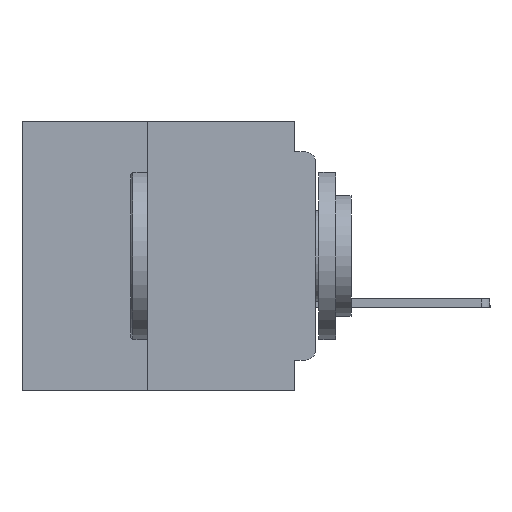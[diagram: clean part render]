
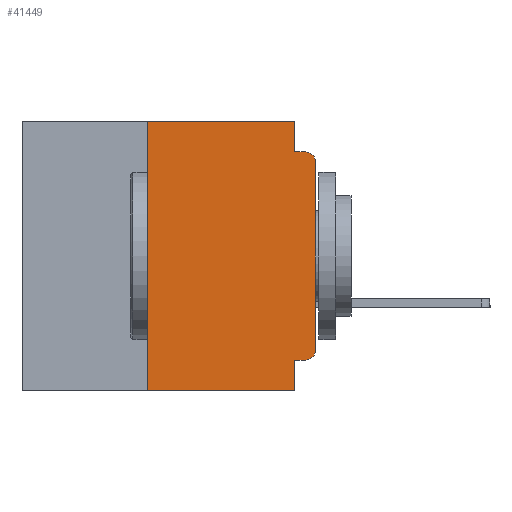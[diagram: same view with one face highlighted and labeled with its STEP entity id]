
A CAD part, left-side view. The second image highlights one B-rep face of the part: STEP entity #41449.
In plain terms, the highlighted planar face has unit normal (-1, 0, 0).
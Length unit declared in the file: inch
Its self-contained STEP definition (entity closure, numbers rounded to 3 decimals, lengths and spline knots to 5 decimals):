
#252 = EDGE_CURVE ( 'NONE', #31251, #6928, #20471, .T. ) ;
#1255 = ORIENTED_EDGE ( 'NONE', *, *, #13003, .T. ) ;
#1754 = CARTESIAN_POINT ( 'NONE',  ( 0., 0.015, -0.06 ) ) ;
#2234 = DIRECTION ( 'NONE',  ( 0., 0., -1. ) ) ;
#2316 = VERTEX_POINT ( 'NONE', #21402 ) ;
#2410 = DIRECTION ( 'NONE',  ( 0., 1., 0. ) ) ;
#2604 = EDGE_CURVE ( 'NONE', #42110, #24186, #23559, .T. ) ;
#3293 = ORIENTED_EDGE ( 'NONE', *, *, #38096, .F. ) ;
#3541 = VECTOR ( 'NONE', #38737, 39.37008 ) ;
#3686 = CARTESIAN_POINT ( 'NONE',  ( 0., 0.031, -0.4 ) ) ;
#4712 = CARTESIAN_POINT ( 'NONE',  ( 0., 0.015, -0.045 ) ) ;
#4891 = CARTESIAN_POINT ( 'NONE',  ( 0., 0.437, 0. ) ) ;
#5028 = CARTESIAN_POINT ( 'NONE',  ( 0., 0.031, -0.4 ) ) ;
#5250 = DIRECTION ( 'NONE',  ( 0., 0., -1. ) ) ;
#6207 = CARTESIAN_POINT ( 'NONE',  ( 0., 0.25, -0.4 ) ) ;
#6416 = VECTOR ( 'NONE', #16457, 39.37008 ) ;
#6928 = VERTEX_POINT ( 'NONE', #34183 ) ;
#7111 = VECTOR ( 'NONE', #31496, 39.37008 ) ;
#8429 = EDGE_CURVE ( 'NONE', #24513, #2316, #20397, .T. ) ;
#9108 = CIRCLE ( 'NONE', #9518, 0.015 ) ;
#9312 = LINE ( 'NONE', #4891, #27503 ) ;
#9518 = AXIS2_PLACEMENT_3D ( 'NONE', #1754, #25774, #5250 ) ;
#10594 = FACE_OUTER_BOUND ( 'NONE', #19734, .T. ) ;
#10923 = VERTEX_POINT ( 'NONE', #41320 ) ;
#11054 = CARTESIAN_POINT ( 'NONE',  ( 0., 0.015, -0.355 ) ) ;
#11506 = CARTESIAN_POINT ( 'NONE',  ( 0., 0.437, -0.4 ) ) ;
#12019 = ORIENTED_EDGE ( 'NONE', *, *, #22201, .F. ) ;
#12280 = VECTOR ( 'NONE', #2410, 39.37008 ) ;
#12559 = ORIENTED_EDGE ( 'NONE', *, *, #2604, .F. ) ;
#12581 = CARTESIAN_POINT ( 'NONE',  ( 0., 0.031, -0.045 ) ) ;
#13003 = EDGE_CURVE ( 'NONE', #22695, #21965, #9108, .T. ) ;
#14071 = CARTESIAN_POINT ( 'NONE',  ( 0., 0.031, 0. ) ) ;
#16457 = DIRECTION ( 'NONE',  ( 0., 0., -1. ) ) ;
#17363 = EDGE_CURVE ( 'NONE', #2316, #22695, #33473, .T. ) ;
#17394 = CARTESIAN_POINT ( 'NONE',  ( 0., 0.031, 0. ) ) ;
#17641 = AXIS2_PLACEMENT_3D ( 'NONE', #43059, #22807, #2234 ) ;
#18652 = DIRECTION ( 'NONE',  ( 0., 0., -1. ) ) ;
#19734 = EDGE_LOOP ( 'NONE', ( #34587, #1255, #3293, #12559, #28935, #22426, #41295, #43618, #12019, #43406 ) ) ;
#20397 = CIRCLE ( 'NONE', #17641, 0.015 ) ;
#20471 = LINE ( 'NONE', #35310, #37473 ) ;
#21402 = CARTESIAN_POINT ( 'NONE',  ( 0., 0., -0.34 ) ) ;
#21423 = LINE ( 'NONE', #39856, #12280 ) ;
#21965 = VERTEX_POINT ( 'NONE', #4712 ) ;
#22201 = EDGE_CURVE ( 'NONE', #24513, #10923, #21423, .T. ) ;
#22426 = ORIENTED_EDGE ( 'NONE', *, *, #252, .F. ) ;
#22695 = VERTEX_POINT ( 'NONE', #39214 ) ;
#22807 = DIRECTION ( 'NONE',  ( -1., 0., 0. ) ) ;
#23559 = LINE ( 'NONE', #17394, #6416 ) ;
#23579 = DIRECTION ( 'NONE',  ( 0., 0., -1. ) ) ;
#24186 = VERTEX_POINT ( 'NONE', #12581 ) ;
#24513 = VERTEX_POINT ( 'NONE', #11054 ) ;
#24679 = CARTESIAN_POINT ( 'NONE',  ( 0., 0., -0.045 ) ) ;
#25773 = CARTESIAN_POINT ( 'NONE',  ( 0., 0., 0. ) ) ;
#25774 = DIRECTION ( 'NONE',  ( -1., 0., 0. ) ) ;
#27082 = VECTOR ( 'NONE', #18652, 39.37008 ) ;
#27503 = VECTOR ( 'NONE', #28817, 39.37008 ) ;
#27738 = VERTEX_POINT ( 'NONE', #3686 ) ;
#28123 = LINE ( 'NONE', #5028, #27082 ) ;
#28817 = DIRECTION ( 'NONE',  ( 0., -1., 0. ) ) ;
#28935 = ORIENTED_EDGE ( 'NONE', *, *, #37202, .F. ) ;
#31251 = VERTEX_POINT ( 'NONE', #6207 ) ;
#31366 = VECTOR ( 'NONE', #35962, 39.37008 ) ;
#31496 = DIRECTION ( 'NONE',  ( 0., -1., 0. ) ) ;
#31852 = LINE ( 'NONE', #11506, #3541 ) ;
#33473 = LINE ( 'NONE', #25773, #31366 ) ;
#33952 = DIRECTION ( 'NONE',  ( 0., 0., 1. ) ) ;
#34183 = CARTESIAN_POINT ( 'NONE',  ( 0., 0.25, 0. ) ) ;
#34286 = LINE ( 'NONE', #24679, #7111 ) ;
#34587 = ORIENTED_EDGE ( 'NONE', *, *, #17363, .T. ) ;
#35310 = CARTESIAN_POINT ( 'NONE',  ( 0., 0.25, -0.4 ) ) ;
#35501 = EDGE_CURVE ( 'NONE', #10923, #27738, #28123, .T. ) ;
#35962 = DIRECTION ( 'NONE',  ( 0., 0., 1. ) ) ;
#37044 = CARTESIAN_POINT ( 'NONE',  ( 0., 0.437, 0. ) ) ;
#37202 = EDGE_CURVE ( 'NONE', #6928, #42110, #9312, .T. ) ;
#37473 = VECTOR ( 'NONE', #33952, 39.37008 ) ;
#38096 = EDGE_CURVE ( 'NONE', #24186, #21965, #34286, .T. ) ;
#38279 = AXIS2_PLACEMENT_3D ( 'NONE', #37044, #43834, #23579 ) ;
#38737 = DIRECTION ( 'NONE',  ( 0., -1., 0. ) ) ;
#39214 = CARTESIAN_POINT ( 'NONE',  ( 0., 0., -0.06 ) ) ;
#39856 = CARTESIAN_POINT ( 'NONE',  ( 0., 0., -0.355 ) ) ;
#40423 = PLANE ( 'NONE',  #38279 ) ;
#41295 = ORIENTED_EDGE ( 'NONE', *, *, #42292, .T. ) ;
#41320 = CARTESIAN_POINT ( 'NONE',  ( 0., 0.031, -0.355 ) ) ;
#41449 = ADVANCED_FACE ( 'NONE', ( #10594 ), #40423, .F. ) ;
#42110 = VERTEX_POINT ( 'NONE', #14071 ) ;
#42292 = EDGE_CURVE ( 'NONE', #31251, #27738, #31852, .T. ) ;
#43059 = CARTESIAN_POINT ( 'NONE',  ( 0., 0.015, -0.34 ) ) ;
#43406 = ORIENTED_EDGE ( 'NONE', *, *, #8429, .T. ) ;
#43618 = ORIENTED_EDGE ( 'NONE', *, *, #35501, .F. ) ;
#43834 = DIRECTION ( 'NONE',  ( 1., 0., 0. ) ) ;
